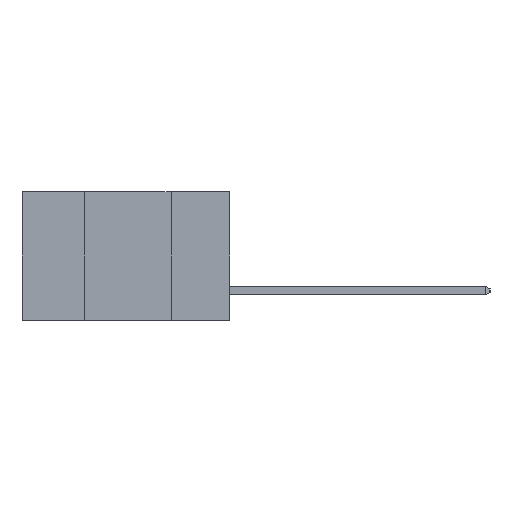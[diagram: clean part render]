
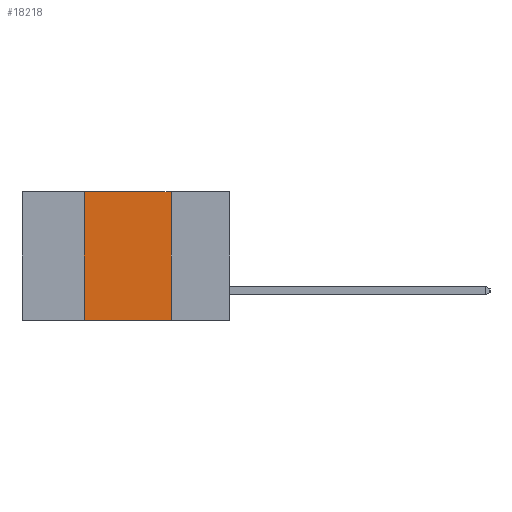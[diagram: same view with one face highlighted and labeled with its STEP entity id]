
A CAD part, left-side view. The second image highlights one B-rep face of the part: STEP entity #18218.
In plain terms, the highlighted planar face has unit normal (-1, 0, 0).
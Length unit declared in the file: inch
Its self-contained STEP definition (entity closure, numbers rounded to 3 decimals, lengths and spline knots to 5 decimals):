
#649 = DIRECTION ( 'NONE',  ( 0., -1., 0. ) ) ;
#673 = EDGE_CURVE ( 'NONE', #13853, #9468, #9287, .T. ) ;
#1673 = CARTESIAN_POINT ( 'NONE',  ( 0., 0.6, 0. ) ) ;
#2966 = EDGE_CURVE ( 'NONE', #8279, #9468, #19980, .T. ) ;
#3269 = DIRECTION ( 'NONE',  ( 0., 0., 1. ) ) ;
#5875 = VECTOR ( 'NONE', #649, 39.37008 ) ;
#6916 = ORIENTED_EDGE ( 'NONE', *, *, #673, .F. ) ;
#6987 = CARTESIAN_POINT ( 'NONE',  ( 0., 0.42, 0. ) ) ;
#7437 = ORIENTED_EDGE ( 'NONE', *, *, #7904, .F. ) ;
#7904 = EDGE_CURVE ( 'NONE', #20857, #13853, #10312, .T. ) ;
#7955 = ORIENTED_EDGE ( 'NONE', *, *, #20575, .F. ) ;
#8279 = VERTEX_POINT ( 'NONE', #14593 ) ;
#8611 = CARTESIAN_POINT ( 'NONE',  ( 0., 0.17, 0. ) ) ;
#9287 = LINE ( 'NONE', #8611, #13034 ) ;
#9404 = FACE_OUTER_BOUND ( 'NONE', #12292, .T. ) ;
#9451 = CARTESIAN_POINT ( 'NONE',  ( 0., 0.6, -0.37 ) ) ;
#9468 = VERTEX_POINT ( 'NONE', #10751 ) ;
#9897 = DIRECTION ( 'NONE',  ( 0., -1., 0. ) ) ;
#10120 = AXIS2_PLACEMENT_3D ( 'NONE', #17979, #19543, #10208 ) ;
#10208 = DIRECTION ( 'NONE',  ( 0., 0., -1. ) ) ;
#10312 = LINE ( 'NONE', #1673, #5875 ) ;
#10751 = CARTESIAN_POINT ( 'NONE',  ( 0., 0.17, -0.37 ) ) ;
#11574 = CARTESIAN_POINT ( 'NONE',  ( 0., 0.42, 0. ) ) ;
#12292 = EDGE_LOOP ( 'NONE', ( #6916, #7437, #7955, #12781 ) ) ;
#12781 = ORIENTED_EDGE ( 'NONE', *, *, #2966, .T. ) ;
#13034 = VECTOR ( 'NONE', #14693, 39.37008 ) ;
#13853 = VERTEX_POINT ( 'NONE', #17548 ) ;
#14593 = CARTESIAN_POINT ( 'NONE',  ( 0., 0.42, -0.37 ) ) ;
#14693 = DIRECTION ( 'NONE',  ( 0., 0., -1. ) ) ;
#15768 = VECTOR ( 'NONE', #3269, 39.37008 ) ;
#16422 = PLANE ( 'NONE',  #10120 ) ;
#16729 = LINE ( 'NONE', #11574, #15768 ) ;
#17548 = CARTESIAN_POINT ( 'NONE',  ( 0., 0.17, 0. ) ) ;
#17979 = CARTESIAN_POINT ( 'NONE',  ( 0., 0.6, 0. ) ) ;
#18218 = ADVANCED_FACE ( 'NONE', ( #9404 ), #16422, .F. ) ;
#19514 = VECTOR ( 'NONE', #9897, 39.37008 ) ;
#19543 = DIRECTION ( 'NONE',  ( 1., 0., 0. ) ) ;
#19980 = LINE ( 'NONE', #9451, #19514 ) ;
#20575 = EDGE_CURVE ( 'NONE', #8279, #20857, #16729, .T. ) ;
#20857 = VERTEX_POINT ( 'NONE', #6987 ) ;
